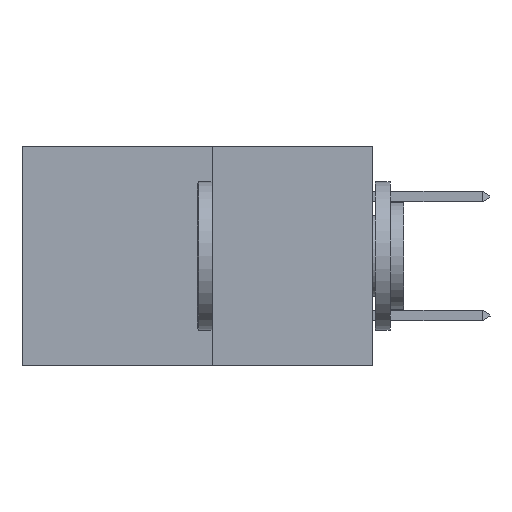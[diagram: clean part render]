
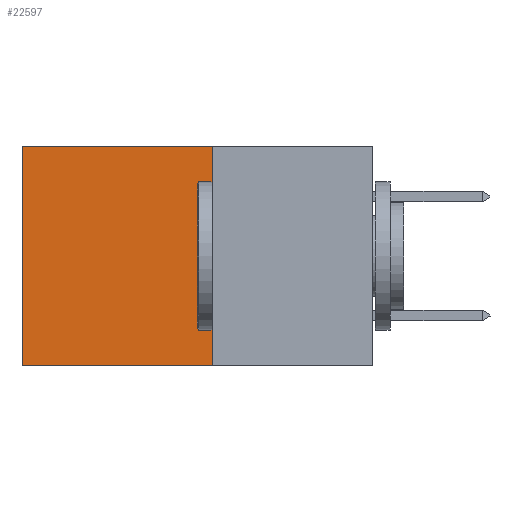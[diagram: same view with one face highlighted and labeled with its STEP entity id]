
A CAD part, left-side view. The second image highlights one B-rep face of the part: STEP entity #22597.
In plain terms, the highlighted planar face has unit normal (-1, 0, 0).
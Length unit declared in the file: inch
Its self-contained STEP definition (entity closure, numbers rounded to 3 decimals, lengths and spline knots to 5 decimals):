
#1697 = PLANE ( 'NONE',  #22763 ) ;
#1978 = ORIENTED_EDGE ( 'NONE', *, *, #7732, .T. ) ;
#4101 = DIRECTION ( 'NONE',  ( 0., 0., -1. ) ) ;
#5062 = EDGE_CURVE ( 'NONE', #25633, #28519, #25783, .T. ) ;
#6763 = VECTOR ( 'NONE', #15211, 39.37008 ) ;
#7370 = CARTESIAN_POINT ( 'NONE',  ( 0.277, 0.27, -0.37 ) ) ;
#7556 = EDGE_CURVE ( 'NONE', #25633, #14064, #25679, .T. ) ;
#7732 = EDGE_CURVE ( 'NONE', #14064, #13710, #21949, .T. ) ;
#11083 = ORIENTED_EDGE ( 'NONE', *, *, #7556, .T. ) ;
#11219 = CARTESIAN_POINT ( 'NONE',  ( 0.277, 0.59, -0.37 ) ) ;
#12967 = VECTOR ( 'NONE', #17764, 39.37008 ) ;
#13710 = VERTEX_POINT ( 'NONE', #11219 ) ;
#14064 = VERTEX_POINT ( 'NONE', #27237 ) ;
#15211 = DIRECTION ( 'NONE',  ( 0., 0., -1. ) ) ;
#15481 = ORIENTED_EDGE ( 'NONE', *, *, #5062, .F. ) ;
#15493 = DIRECTION ( 'NONE',  ( 0., 0., -1. ) ) ;
#15529 = CARTESIAN_POINT ( 'NONE',  ( 0.277, 0.59, -0.37 ) ) ;
#16100 = CARTESIAN_POINT ( 'NONE',  ( 0.277, 0.27, -0.37 ) ) ;
#17761 = CARTESIAN_POINT ( 'NONE',  ( 0.277, 0.27, 0. ) ) ;
#17764 = DIRECTION ( 'NONE',  ( 0., 1., 0. ) ) ;
#18349 = DIRECTION ( 'NONE',  ( 1., 0., 0. ) ) ;
#18610 = FACE_OUTER_BOUND ( 'NONE', #26835, .T. ) ;
#20428 = VECTOR ( 'NONE', #15493, 39.37008 ) ;
#21509 = EDGE_CURVE ( 'NONE', #28519, #13710, #30732, .T. ) ;
#21747 = CARTESIAN_POINT ( 'NONE',  ( 0.277, 0.27, 0. ) ) ;
#21949 = LINE ( 'NONE', #15529, #20428 ) ;
#22597 = ADVANCED_FACE ( 'NONE', ( #18610 ), #1697, .F. ) ;
#22763 = AXIS2_PLACEMENT_3D ( 'NONE', #23090, #18349, #4101 ) ;
#23024 = VECTOR ( 'NONE', #28702, 39.37008 ) ;
#23070 = ORIENTED_EDGE ( 'NONE', *, *, #21509, .F. ) ;
#23090 = CARTESIAN_POINT ( 'NONE',  ( 0.277, 0.27, -0.37 ) ) ;
#25633 = VERTEX_POINT ( 'NONE', #21747 ) ;
#25679 = LINE ( 'NONE', #17761, #12967 ) ;
#25783 = LINE ( 'NONE', #16100, #6763 ) ;
#26346 = CARTESIAN_POINT ( 'NONE',  ( 0.277, 0.27, -0.37 ) ) ;
#26835 = EDGE_LOOP ( 'NONE', ( #1978, #23070, #15481, #11083 ) ) ;
#27237 = CARTESIAN_POINT ( 'NONE',  ( 0.277, 0.59, 0. ) ) ;
#28519 = VERTEX_POINT ( 'NONE', #7370 ) ;
#28702 = DIRECTION ( 'NONE',  ( 0., 1., 0. ) ) ;
#30732 = LINE ( 'NONE', #26346, #23024 ) ;
